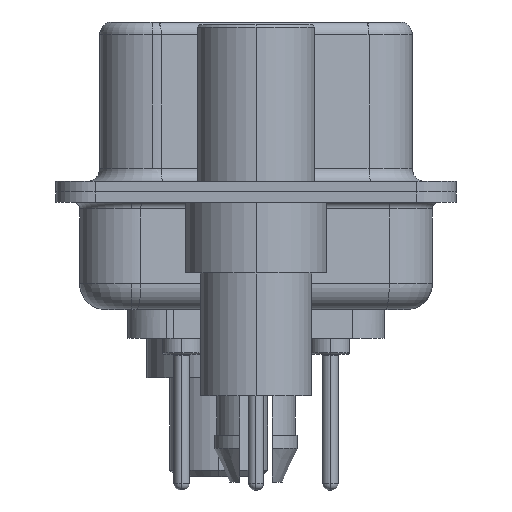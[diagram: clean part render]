
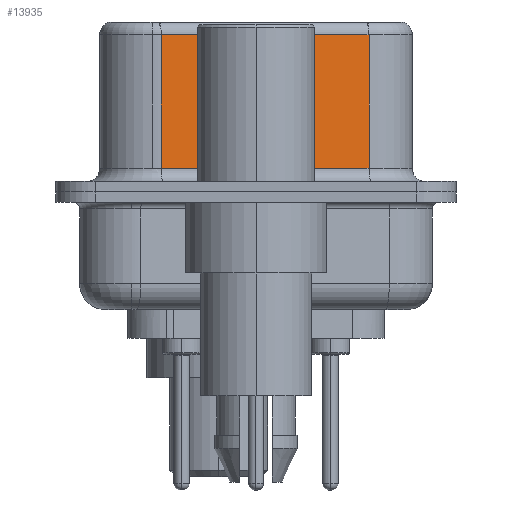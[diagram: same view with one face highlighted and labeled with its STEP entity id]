
A CAD part, left-side view. The second image highlights one B-rep face of the part: STEP entity #13935.
In plain terms, the highlighted planar face has unit normal (-0.985, -0.174, 0).
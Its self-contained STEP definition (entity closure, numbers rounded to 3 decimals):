
#403 = EDGE_CURVE ( 'NONE', #24153, #27073, #6470, .T. ) ;
#1230 = CARTESIAN_POINT ( 'NONE',  ( 3.73, 3.628, 6.02 ) ) ;
#1319 = LINE ( 'NONE', #3542, #1700 ) ;
#1606 = LINE ( 'NONE', #7448, #28662 ) ;
#1700 = VECTOR ( 'NONE', #28559, 1000. ) ;
#3542 = CARTESIAN_POINT ( 'NONE',  ( 5.132, -4.322, 0.9 ) ) ;
#3572 = CARTESIAN_POINT ( 'NONE',  ( 5.132, -4.322, 0.9 ) ) ;
#3984 = VECTOR ( 'NONE', #29239, 1000. ) ;
#4812 = AXIS2_PLACEMENT_3D ( 'NONE', #12711, #19661, #17159 ) ;
#5915 = CARTESIAN_POINT ( 'NONE',  ( 5.132, -4.322, 6.02 ) ) ;
#6320 = DIRECTION ( 'NONE',  ( -0.174, 0.985, 0. ) ) ;
#6374 = ORIENTED_EDGE ( 'NONE', *, *, #403, .T. ) ;
#6470 = LINE ( 'NONE', #19807, #28814 ) ;
#7448 = CARTESIAN_POINT ( 'NONE',  ( 3.73, 3.628, 6.52 ) ) ;
#8316 = CARTESIAN_POINT ( 'NONE',  ( 3.73, 3.628, 0.9 ) ) ;
#8777 = ORIENTED_EDGE ( 'NONE', *, *, #18651, .T. ) ;
#9115 = CARTESIAN_POINT ( 'NONE',  ( 5.132, -4.322, 6.52 ) ) ;
#11111 = EDGE_CURVE ( 'NONE', #24153, #24065, #27038, .T. ) ;
#11980 = DIRECTION ( 'NONE',  ( 0., 0., -1. ) ) ;
#12529 = VERTEX_POINT ( 'NONE', #8316 ) ;
#12711 = CARTESIAN_POINT ( 'NONE',  ( 5.132, -4.322, 6.52 ) ) ;
#13242 = ORIENTED_EDGE ( 'NONE', *, *, #16411, .T. ) ;
#13324 = EDGE_LOOP ( 'NONE', ( #27083, #6374, #13242, #8777 ) ) ;
#13935 = ADVANCED_FACE ( 'NONE', ( #25138 ), #17053, .F. ) ;
#16411 = EDGE_CURVE ( 'NONE', #27073, #12529, #1606, .T. ) ;
#17053 = PLANE ( 'NONE',  #4812 ) ;
#17159 = DIRECTION ( 'NONE',  ( -0.174, 0.985, 0. ) ) ;
#18651 = EDGE_CURVE ( 'NONE', #12529, #24065, #1319, .T. ) ;
#19661 = DIRECTION ( 'NONE',  ( 0.985, 0.174, 0. ) ) ;
#19807 = CARTESIAN_POINT ( 'NONE',  ( 5.132, -4.322, 6.02 ) ) ;
#24065 = VERTEX_POINT ( 'NONE', #3572 ) ;
#24153 = VERTEX_POINT ( 'NONE', #5915 ) ;
#25138 = FACE_OUTER_BOUND ( 'NONE', #13324, .T. ) ;
#27038 = LINE ( 'NONE', #9115, #3984 ) ;
#27073 = VERTEX_POINT ( 'NONE', #1230 ) ;
#27083 = ORIENTED_EDGE ( 'NONE', *, *, #11111, .F. ) ;
#28559 = DIRECTION ( 'NONE',  ( 0.174, -0.985, 0. ) ) ;
#28662 = VECTOR ( 'NONE', #11980, 1000. ) ;
#28814 = VECTOR ( 'NONE', #6320, 1000. ) ;
#29239 = DIRECTION ( 'NONE',  ( 0., 0., -1. ) ) ;
